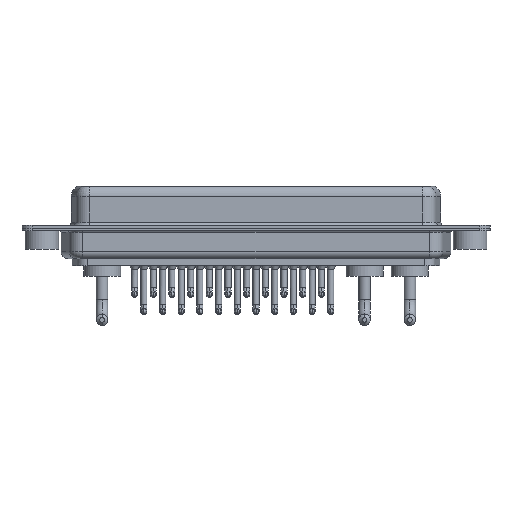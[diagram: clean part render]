
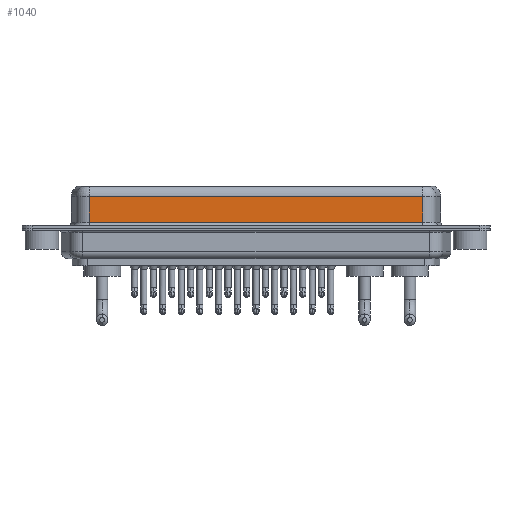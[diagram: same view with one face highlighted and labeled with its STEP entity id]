
A CAD part, front view. The second image highlights one B-rep face of the part: STEP entity #1040.
In plain terms, the highlighted planar face has unit normal (0, -1, 0).
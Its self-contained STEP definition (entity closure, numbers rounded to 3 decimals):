
#274 = DIRECTION ( 'NONE',  ( 0., 1., 0. ) ) ;
#610 = VERTEX_POINT ( 'NONE', #12239 ) ;
#1040 = ADVANCED_FACE ( 'NONE', ( #5670 ), #5437, .F. ) ;
#1279 = DIRECTION ( 'NONE',  ( 0., 0., -1. ) ) ;
#2104 = ORIENTED_EDGE ( 'NONE', *, *, #7159, .T. ) ;
#4264 = VERTEX_POINT ( 'NONE', #6900 ) ;
#4626 = CARTESIAN_POINT ( 'NONE',  ( 56.462, -3.95, 4.65 ) ) ;
#5193 = CARTESIAN_POINT ( 'NONE',  ( 7.038, -3.95, 6.4 ) ) ;
#5437 = PLANE ( 'NONE',  #8744 ) ;
#5670 = FACE_OUTER_BOUND ( 'NONE', #20589, .T. ) ;
#6671 = VECTOR ( 'NONE', #10960, 1000. ) ;
#6900 = CARTESIAN_POINT ( 'NONE',  ( 7.038, -3.95, 4.65 ) ) ;
#6950 = EDGE_CURVE ( 'NONE', #7711, #610, #14225, .T. ) ;
#7159 = EDGE_CURVE ( 'NONE', #8862, #4264, #7809, .T. ) ;
#7346 = CARTESIAN_POINT ( 'NONE',  ( 56.462, -3.95, 0.9 ) ) ;
#7711 = VERTEX_POINT ( 'NONE', #21666 ) ;
#7809 = LINE ( 'NONE', #11558, #14034 ) ;
#8547 = EDGE_CURVE ( 'NONE', #8862, #610, #14681, .T. ) ;
#8744 = AXIS2_PLACEMENT_3D ( 'NONE', #16675, #274, #14863 ) ;
#8862 = VERTEX_POINT ( 'NONE', #4626 ) ;
#9578 = EDGE_CURVE ( 'NONE', #4264, #7711, #23327, .T. ) ;
#9742 = DIRECTION ( 'NONE',  ( -1., 0., 0. ) ) ;
#10960 = DIRECTION ( 'NONE',  ( 1., 0., 0. ) ) ;
#11558 = CARTESIAN_POINT ( 'NONE',  ( 56.462, -3.95, 4.65 ) ) ;
#12239 = CARTESIAN_POINT ( 'NONE',  ( 56.462, -3.95, 0.9 ) ) ;
#14034 = VECTOR ( 'NONE', #9742, 1000. ) ;
#14050 = VECTOR ( 'NONE', #16065, 1000. ) ;
#14225 = LINE ( 'NONE', #7346, #6671 ) ;
#14601 = ORIENTED_EDGE ( 'NONE', *, *, #6950, .T. ) ;
#14681 = LINE ( 'NONE', #16005, #18739 ) ;
#14863 = DIRECTION ( 'NONE',  ( 0., 0., 1. ) ) ;
#16005 = CARTESIAN_POINT ( 'NONE',  ( 56.462, -3.95, 6.4 ) ) ;
#16065 = DIRECTION ( 'NONE',  ( 0., 0., -1. ) ) ;
#16675 = CARTESIAN_POINT ( 'NONE',  ( 56.462, -3.95, 6.4 ) ) ;
#16962 = ORIENTED_EDGE ( 'NONE', *, *, #9578, .T. ) ;
#18739 = VECTOR ( 'NONE', #1279, 1000. ) ;
#20589 = EDGE_LOOP ( 'NONE', ( #22177, #2104, #16962, #14601 ) ) ;
#21666 = CARTESIAN_POINT ( 'NONE',  ( 7.038, -3.95, 0.9 ) ) ;
#22177 = ORIENTED_EDGE ( 'NONE', *, *, #8547, .F. ) ;
#23327 = LINE ( 'NONE', #5193, #14050 ) ;
